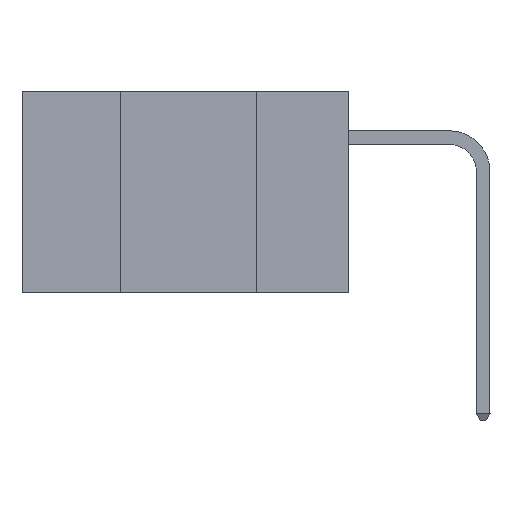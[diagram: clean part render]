
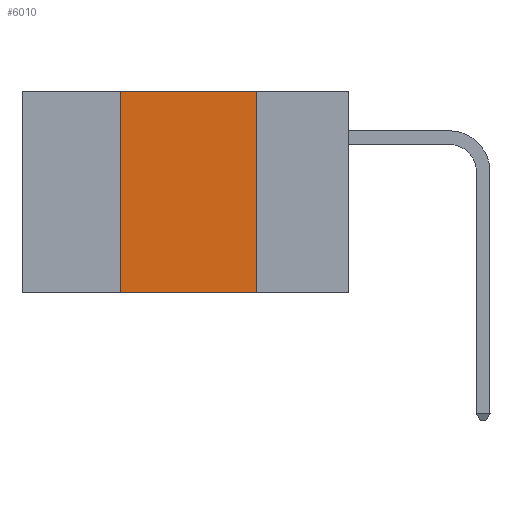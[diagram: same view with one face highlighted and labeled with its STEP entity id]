
A CAD part, left-side view. The second image highlights one B-rep face of the part: STEP entity #6010.
In plain terms, the highlighted planar face has unit normal (-1, 0, 0).
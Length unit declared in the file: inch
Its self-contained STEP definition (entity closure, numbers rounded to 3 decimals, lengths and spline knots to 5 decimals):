
#1832 = CARTESIAN_POINT ( 'NONE',  ( 0., 0.6, 0. ) ) ;
#2317 = EDGE_LOOP ( 'NONE', ( #40771, #17686, #8065, #15066 ) ) ;
#3730 = EDGE_CURVE ( 'NONE', #9580, #26758, #42237, .T. ) ;
#4436 = FACE_OUTER_BOUND ( 'NONE', #2317, .T. ) ;
#4750 = VERTEX_POINT ( 'NONE', #12711 ) ;
#4874 = LINE ( 'NONE', #37950, #35854 ) ;
#6010 = ADVANCED_FACE ( 'NONE', ( #4436 ), #31453, .F. ) ;
#8065 = ORIENTED_EDGE ( 'NONE', *, *, #35965, .F. ) ;
#9063 = VECTOR ( 'NONE', #12377, 39.37008 ) ;
#9580 = VERTEX_POINT ( 'NONE', #25843 ) ;
#12377 = DIRECTION ( 'NONE',  ( 0., 0., 1. ) ) ;
#12711 = CARTESIAN_POINT ( 'NONE',  ( 0., 0.42, 0. ) ) ;
#15036 = DIRECTION ( 'NONE',  ( 1., 0., 0. ) ) ;
#15066 = ORIENTED_EDGE ( 'NONE', *, *, #3730, .T. ) ;
#16713 = DIRECTION ( 'NONE',  ( 0., -1., 0. ) ) ;
#17686 = ORIENTED_EDGE ( 'NONE', *, *, #33128, .F. ) ;
#18201 = CARTESIAN_POINT ( 'NONE',  ( 0., 0.42, 0. ) ) ;
#20825 = CARTESIAN_POINT ( 'NONE',  ( 0., 0.6, 0. ) ) ;
#24555 = AXIS2_PLACEMENT_3D ( 'NONE', #1832, #15036, #41420 ) ;
#25541 = VECTOR ( 'NONE', #31848, 39.37008 ) ;
#25843 = CARTESIAN_POINT ( 'NONE',  ( 0., 0.42, -0.37 ) ) ;
#26758 = VERTEX_POINT ( 'NONE', #28592 ) ;
#28421 = DIRECTION ( 'NONE',  ( 0., 0., -1. ) ) ;
#28592 = CARTESIAN_POINT ( 'NONE',  ( 0., 0.17, -0.37 ) ) ;
#31453 = PLANE ( 'NONE',  #24555 ) ;
#31848 = DIRECTION ( 'NONE',  ( 0., -1., 0. ) ) ;
#32050 = CARTESIAN_POINT ( 'NONE',  ( 0., 0.6, -0.37 ) ) ;
#33128 = EDGE_CURVE ( 'NONE', #4750, #37558, #34001, .T. ) ;
#34001 = LINE ( 'NONE', #20825, #37181 ) ;
#34028 = EDGE_CURVE ( 'NONE', #37558, #26758, #4874, .T. ) ;
#34388 = CARTESIAN_POINT ( 'NONE',  ( 0., 0.17, 0. ) ) ;
#35854 = VECTOR ( 'NONE', #28421, 39.37008 ) ;
#35965 = EDGE_CURVE ( 'NONE', #9580, #4750, #41999, .T. ) ;
#37181 = VECTOR ( 'NONE', #16713, 39.37008 ) ;
#37558 = VERTEX_POINT ( 'NONE', #34388 ) ;
#37950 = CARTESIAN_POINT ( 'NONE',  ( 0., 0.17, 0. ) ) ;
#40771 = ORIENTED_EDGE ( 'NONE', *, *, #34028, .F. ) ;
#41420 = DIRECTION ( 'NONE',  ( 0., 0., -1. ) ) ;
#41999 = LINE ( 'NONE', #18201, #9063 ) ;
#42237 = LINE ( 'NONE', #32050, #25541 ) ;
